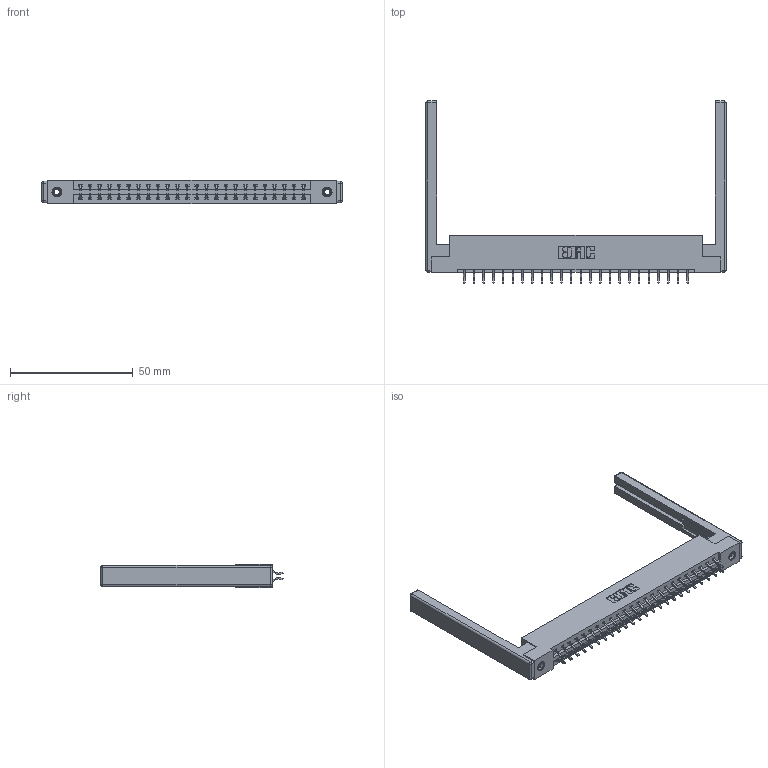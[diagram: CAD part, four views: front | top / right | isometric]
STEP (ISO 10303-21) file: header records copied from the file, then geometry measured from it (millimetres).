
FILE_DESCRIPTION (( 'STEP AP203' ), '1' );
FILE_NAME ('337-048-556-268.STEP', '2019-10-09T15:10:17', ( '' ), ( '' ), 'SwSTEP 2.0', 'SolidWorks 2016', '' );
FILE_SCHEMA (( 'CONFIG_CONTROL_DESIGN' ));
Length unit declared in the file: inch
Products named in the file (5): 307-220-068; 337 Part_Flush Mounting Lugs - 0.156 Dia-TI; 337-048-556-268; 345-250-001_345-250-001-102; 345-292-001_556 Tail
Assembly tree (53 placements, depth 2):
  337-048-556-268
    337 Part_Flush Mounting Lugs - 0.156 Dia-TI
    345-292-001_556 Tail  x48
    345-250-001_345-250-001-102  x2
    307-220-068  x2
Bounding box: 122.53 x 74.31 x 9.4 mm (x, y, z)
Volume: 17056.4 mm3; surface area: 18134.2 mm2
Topology: 53 solids, 53 shells, 3148 faces, 9293 edges, 6110 vertices
Faces by surface type: plane 2174, cylinder 950, cone 12, sphere 8, torus 4
Entity records: 23916 total; most frequent: CARTESIAN_POINT 4023, ORIENTED_EDGE 3936, DIRECTION 3514, EDGE_CURVE 1968, VECTOR 1782, LINE 1782, VERTEX_POINT 1302, AXIS2_PLACEMENT_3D 866
